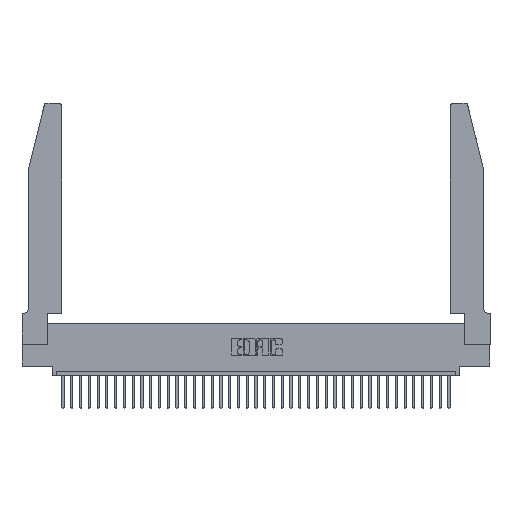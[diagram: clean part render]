
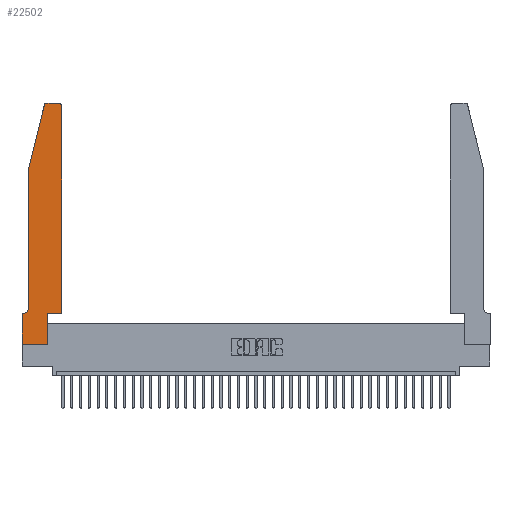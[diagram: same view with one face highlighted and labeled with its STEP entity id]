
A CAD part, top view. The second image highlights one B-rep face of the part: STEP entity #22502.
In plain terms, the highlighted planar face has unit normal (0, 0, 1).
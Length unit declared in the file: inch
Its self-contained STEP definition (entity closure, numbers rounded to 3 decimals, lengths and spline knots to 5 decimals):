
#682 = CARTESIAN_POINT ( 'NONE',  ( 0.0055, 0.42, 0.37 ) ) ;
#1243 = DIRECTION ( 'NONE',  ( -0.239, -0.971, 0. ) ) ;
#1262 = CARTESIAN_POINT ( 'NONE',  ( 0., 0., 0.37 ) ) ;
#1952 = EDGE_CURVE ( 'NONE', #9619, #12059, #23900, .T. ) ;
#2045 = CARTESIAN_POINT ( 'NONE',  ( 0.4505, 0.35, 0.37 ) ) ;
#2338 = EDGE_CURVE ( 'NONE', #10875, #26529, #37273, .T. ) ;
#3459 = AXIS2_PLACEMENT_3D ( 'NONE', #25661, #37410, #34348 ) ;
#3736 = DIRECTION ( 'NONE',  ( -1., 0., 0. ) ) ;
#5133 = EDGE_CURVE ( 'NONE', #35431, #20219, #38038, .T. ) ;
#6183 = CARTESIAN_POINT ( 'NONE',  ( 0.2865, 0.35, 0.37 ) ) ;
#6239 = ORIENTED_EDGE ( 'NONE', *, *, #6997, .T. ) ;
#6494 = CARTESIAN_POINT ( 'NONE',  ( 0.2865, 0., 0.37 ) ) ;
#6675 = DIRECTION ( 'NONE',  ( 0., 0., 1. ) ) ;
#6895 = CIRCLE ( 'NONE', #12138, 0.03 ) ;
#6997 = EDGE_CURVE ( 'NONE', #8621, #8555, #31513, .T. ) ;
#7094 = VECTOR ( 'NONE', #1243, 39.37008 ) ;
#7108 = DIRECTION ( 'NONE',  ( 0., -1., 0. ) ) ;
#7307 = CARTESIAN_POINT ( 'NONE',  ( 0.284, 2.75, 0.37 ) ) ;
#8109 = DIRECTION ( 'NONE',  ( 1., 0., 0. ) ) ;
#8555 = VERTEX_POINT ( 'NONE', #27663 ) ;
#8621 = VERTEX_POINT ( 'NONE', #10127 ) ;
#9168 = CARTESIAN_POINT ( 'NONE',  ( 0.2865, 0.35, 0.37 ) ) ;
#9609 = CIRCLE ( 'NONE', #3459, 0.03 ) ;
#9619 = VERTEX_POINT ( 'NONE', #1262 ) ;
#10127 = CARTESIAN_POINT ( 'NONE',  ( 0.4505, 0.35, 0.37 ) ) ;
#10538 = CARTESIAN_POINT ( 'NONE',  ( 0.0755, 2., 0.37 ) ) ;
#10674 = VECTOR ( 'NONE', #12985, 39.37008 ) ;
#10875 = VERTEX_POINT ( 'NONE', #24398 ) ;
#11173 = ORIENTED_EDGE ( 'NONE', *, *, #5133, .T. ) ;
#12059 = VERTEX_POINT ( 'NONE', #6494 ) ;
#12138 = AXIS2_PLACEMENT_3D ( 'NONE', #24444, #6675, #12628 ) ;
#12251 = DIRECTION ( 'NONE',  ( 0., 1., 0. ) ) ;
#12278 = CARTESIAN_POINT ( 'NONE',  ( 0.0755, 0.35, 0.37 ) ) ;
#12555 = VERTEX_POINT ( 'NONE', #9168 ) ;
#12628 = DIRECTION ( 'NONE',  ( 1., 0., 0. ) ) ;
#12985 = DIRECTION ( 'NONE',  ( -1., 0., 0. ) ) ;
#13104 = CARTESIAN_POINT ( 'NONE',  ( 0.0755, 2., 0.37 ) ) ;
#14129 = DIRECTION ( 'NONE',  ( 0., 0., 1. ) ) ;
#14583 = ORIENTED_EDGE ( 'NONE', *, *, #16373, .T. ) ;
#16362 = AXIS2_PLACEMENT_3D ( 'NONE', #682, #30542, #18690 ) ;
#16373 = EDGE_CURVE ( 'NONE', #24165, #24160, #36359, .T. ) ;
#16711 = LINE ( 'NONE', #6183, #23248 ) ;
#18251 = CARTESIAN_POINT ( 'NONE',  ( 0.0755, 2., 0.37 ) ) ;
#18320 = VECTOR ( 'NONE', #7108, 39.37008 ) ;
#18690 = DIRECTION ( 'NONE',  ( -1., 0., 0. ) ) ;
#19064 = DIRECTION ( 'NONE',  ( 0., -1., 0. ) ) ;
#19515 = ORIENTED_EDGE ( 'NONE', *, *, #1952, .T. ) ;
#19659 = ORIENTED_EDGE ( 'NONE', *, *, #33904, .T. ) ;
#19779 = EDGE_CURVE ( 'NONE', #24160, #10875, #24195, .T. ) ;
#19909 = DIRECTION ( 'NONE',  ( 0., 1., 0. ) ) ;
#20219 = VERTEX_POINT ( 'NONE', #7307 ) ;
#20979 = EDGE_CURVE ( 'NONE', #20219, #33939, #6895, .T. ) ;
#21940 = DIRECTION ( 'NONE',  ( 1., 0., 0. ) ) ;
#22276 = EDGE_CURVE ( 'NONE', #8555, #35431, #9609, .T. ) ;
#22498 = VECTOR ( 'NONE', #19064, 39.37008 ) ;
#22502 = ADVANCED_FACE ( 'NONE', ( #35109 ), #26296, .T. ) ;
#23239 = CARTESIAN_POINT ( 'NONE',  ( 0., 0., 0.37 ) ) ;
#23248 = VECTOR ( 'NONE', #12251, 39.37008 ) ;
#23322 = EDGE_LOOP ( 'NONE', ( #11173, #34301, #30819, #14583, #35684, #35567, #34425, #19515, #33971, #19659, #6239, #34924 ) ) ;
#23333 = EDGE_CURVE ( 'NONE', #26529, #9619, #34115, .T. ) ;
#23369 = DIRECTION ( 'NONE',  ( 1., 0., 0. ) ) ;
#23900 = LINE ( 'NONE', #23239, #34101 ) ;
#24054 = VECTOR ( 'NONE', #19909, 39.37008 ) ;
#24160 = VERTEX_POINT ( 'NONE', #26809 ) ;
#24165 = VERTEX_POINT ( 'NONE', #18251 ) ;
#24195 = CIRCLE ( 'NONE', #16362, 0.07 ) ;
#24398 = CARTESIAN_POINT ( 'NONE',  ( 0.0055, 0.35, 0.37 ) ) ;
#24444 = CARTESIAN_POINT ( 'NONE',  ( 0.284, 2.72, 0.37 ) ) ;
#25640 = CARTESIAN_POINT ( 'NONE',  ( 0.4505, 0.35, 0.37 ) ) ;
#25661 = CARTESIAN_POINT ( 'NONE',  ( 0.4205, 2.72, 0.37 ) ) ;
#26296 = PLANE ( 'NONE',  #26587 ) ;
#26419 = CARTESIAN_POINT ( 'NONE',  ( 0., 0.35, 0.37 ) ) ;
#26529 = VERTEX_POINT ( 'NONE', #31038 ) ;
#26587 = AXIS2_PLACEMENT_3D ( 'NONE', #26419, #14129, #21940 ) ;
#26675 = LINE ( 'NONE', #2045, #35544 ) ;
#26809 = CARTESIAN_POINT ( 'NONE',  ( 0.0755, 0.42, 0.37 ) ) ;
#27663 = CARTESIAN_POINT ( 'NONE',  ( 0.4505, 2.72, 0.37 ) ) ;
#28902 = CARTESIAN_POINT ( 'NONE',  ( 0.25487, 2.72718, 0.37 ) ) ;
#29640 = EDGE_CURVE ( 'NONE', #33939, #24165, #31242, .T. ) ;
#30542 = DIRECTION ( 'NONE',  ( 0., 0., -1. ) ) ;
#30789 = CARTESIAN_POINT ( 'NONE',  ( 0.2605, 2.75, 0.37 ) ) ;
#30819 = ORIENTED_EDGE ( 'NONE', *, *, #29640, .T. ) ;
#31038 = CARTESIAN_POINT ( 'NONE',  ( 0., 0.35, 0.37 ) ) ;
#31242 = LINE ( 'NONE', #10538, #7094 ) ;
#31513 = LINE ( 'NONE', #25640, #24054 ) ;
#31735 = CARTESIAN_POINT ( 'NONE',  ( 0.4205, 2.75, 0.37 ) ) ;
#33904 = EDGE_CURVE ( 'NONE', #12555, #8621, #26675, .T. ) ;
#33939 = VERTEX_POINT ( 'NONE', #28902 ) ;
#33971 = ORIENTED_EDGE ( 'NONE', *, *, #36740, .T. ) ;
#34101 = VECTOR ( 'NONE', #23369, 39.37008 ) ;
#34115 = LINE ( 'NONE', #36888, #18320 ) ;
#34301 = ORIENTED_EDGE ( 'NONE', *, *, #20979, .T. ) ;
#34348 = DIRECTION ( 'NONE',  ( 1., 0., 0. ) ) ;
#34425 = ORIENTED_EDGE ( 'NONE', *, *, #23333, .T. ) ;
#34924 = ORIENTED_EDGE ( 'NONE', *, *, #22276, .T. ) ;
#35109 = FACE_OUTER_BOUND ( 'NONE', #23322, .T. ) ;
#35431 = VERTEX_POINT ( 'NONE', #31735 ) ;
#35544 = VECTOR ( 'NONE', #8109, 39.37008 ) ;
#35567 = ORIENTED_EDGE ( 'NONE', *, *, #2338, .T. ) ;
#35684 = ORIENTED_EDGE ( 'NONE', *, *, #19779, .T. ) ;
#36351 = VECTOR ( 'NONE', #3736, 39.37008 ) ;
#36359 = LINE ( 'NONE', #13104, #22498 ) ;
#36740 = EDGE_CURVE ( 'NONE', #12059, #12555, #16711, .T. ) ;
#36888 = CARTESIAN_POINT ( 'NONE',  ( 0., 0., 0.37 ) ) ;
#37273 = LINE ( 'NONE', #12278, #36351 ) ;
#37410 = DIRECTION ( 'NONE',  ( 0., 0., 1. ) ) ;
#38038 = LINE ( 'NONE', #30789, #10674 ) ;
